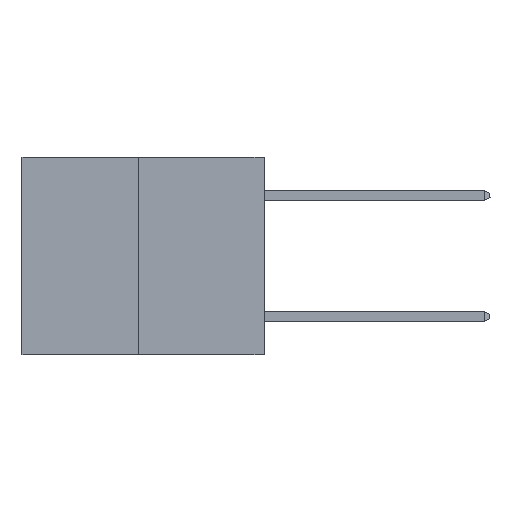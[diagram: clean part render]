
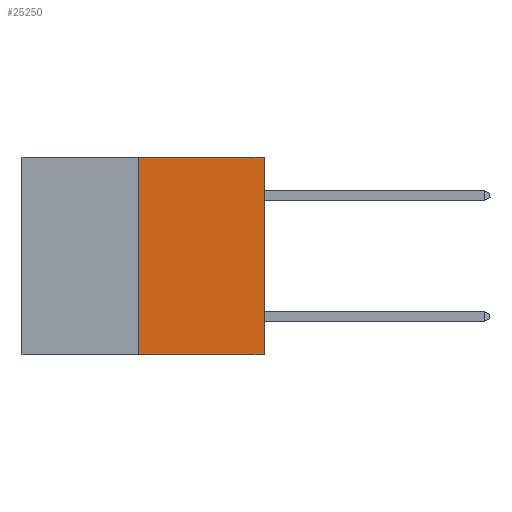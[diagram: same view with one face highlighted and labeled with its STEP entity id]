
A CAD part, left-side view. The second image highlights one B-rep face of the part: STEP entity #25250.
In plain terms, the highlighted planar face has unit normal (-1, 0, 0).
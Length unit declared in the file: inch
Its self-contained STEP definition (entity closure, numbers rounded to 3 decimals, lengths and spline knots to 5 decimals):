
#26 = CARTESIAN_POINT ( 'NONE',  ( 0., 0.312, 0. ) ) ;
#665 = EDGE_LOOP ( 'NONE', ( #12556, #1977, #6852, #18664 ) ) ;
#831 = VECTOR ( 'NONE', #30119, 39.37008 ) ;
#1977 = ORIENTED_EDGE ( 'NONE', *, *, #19622, .T. ) ;
#3191 = EDGE_CURVE ( 'NONE', #7514, #23336, #27905, .T. ) ;
#4465 = VECTOR ( 'NONE', #24575, 39.37008 ) ;
#4621 = EDGE_CURVE ( 'NONE', #23336, #13952, #20116, .T. ) ;
#5750 = FACE_OUTER_BOUND ( 'NONE', #665, .T. ) ;
#6852 = ORIENTED_EDGE ( 'NONE', *, *, #29026, .T. ) ;
#7514 = VERTEX_POINT ( 'NONE', #21183 ) ;
#7599 = DIRECTION ( 'NONE',  ( 0., 0., 1. ) ) ;
#8050 = CARTESIAN_POINT ( 'NONE',  ( 0., 0.312, -0.49 ) ) ;
#11068 = LINE ( 'NONE', #19628, #4465 ) ;
#12357 = CARTESIAN_POINT ( 'NONE',  ( 0., 0., 0. ) ) ;
#12556 = ORIENTED_EDGE ( 'NONE', *, *, #3191, .F. ) ;
#12958 = VERTEX_POINT ( 'NONE', #30085 ) ;
#13813 = CARTESIAN_POINT ( 'NONE',  ( 0., 0., 0. ) ) ;
#13952 = VERTEX_POINT ( 'NONE', #13813 ) ;
#16625 = AXIS2_PLACEMENT_3D ( 'NONE', #21559, #19063, #31304 ) ;
#18664 = ORIENTED_EDGE ( 'NONE', *, *, #4621, .F. ) ;
#19063 = DIRECTION ( 'NONE',  ( 1., 0., 0. ) ) ;
#19622 = EDGE_CURVE ( 'NONE', #7514, #12958, #11068, .T. ) ;
#19628 = CARTESIAN_POINT ( 'NONE',  ( 0., 0.6, -0.49 ) ) ;
#20116 = LINE ( 'NONE', #20124, #831 ) ;
#20124 = CARTESIAN_POINT ( 'NONE',  ( 0., 0.6, 0. ) ) ;
#20584 = DIRECTION ( 'NONE',  ( 0., 0., 1. ) ) ;
#21183 = CARTESIAN_POINT ( 'NONE',  ( 0., 0.312, -0.49 ) ) ;
#21559 = CARTESIAN_POINT ( 'NONE',  ( 0., 0.6, 0. ) ) ;
#22144 = VECTOR ( 'NONE', #20584, 39.37008 ) ;
#23336 = VERTEX_POINT ( 'NONE', #26 ) ;
#24388 = VECTOR ( 'NONE', #7599, 39.37008 ) ;
#24575 = DIRECTION ( 'NONE',  ( 0., -1., 0. ) ) ;
#25250 = ADVANCED_FACE ( 'NONE', ( #5750 ), #28953, .F. ) ;
#27905 = LINE ( 'NONE', #8050, #22144 ) ;
#28953 = PLANE ( 'NONE',  #16625 ) ;
#29026 = EDGE_CURVE ( 'NONE', #12958, #13952, #30907, .T. ) ;
#30085 = CARTESIAN_POINT ( 'NONE',  ( 0., 0., -0.49 ) ) ;
#30119 = DIRECTION ( 'NONE',  ( 0., -1., 0. ) ) ;
#30907 = LINE ( 'NONE', #12357, #24388 ) ;
#31304 = DIRECTION ( 'NONE',  ( 0., 0., -1. ) ) ;
